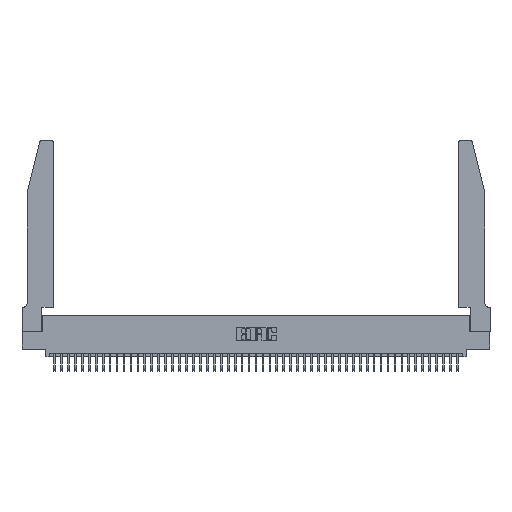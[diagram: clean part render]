
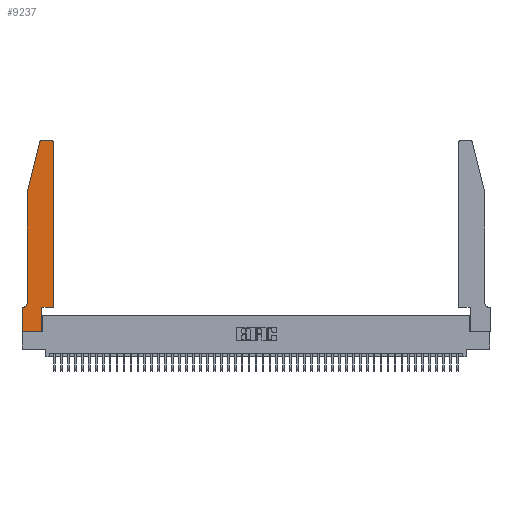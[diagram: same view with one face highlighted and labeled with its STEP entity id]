
A CAD part, top view. The second image highlights one B-rep face of the part: STEP entity #9237.
In plain terms, the highlighted planar face has unit normal (0, 0, 1).
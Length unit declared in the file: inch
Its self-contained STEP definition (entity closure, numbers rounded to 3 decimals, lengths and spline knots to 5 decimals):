
#523 = CARTESIAN_POINT ( 'NONE',  ( 0.25487, 2.72718, 0.37 ) ) ;
#570 = VECTOR ( 'NONE', #8482, 39.37008 ) ;
#900 = AXIS2_PLACEMENT_3D ( 'NONE', #37943, #14692, #41812 ) ;
#2733 = CARTESIAN_POINT ( 'NONE',  ( 0.2865, 0.35, 0.37 ) ) ;
#3807 = VERTEX_POINT ( 'NONE', #523 ) ;
#3835 = DIRECTION ( 'NONE',  ( -1., 0., 0. ) ) ;
#4139 = CARTESIAN_POINT ( 'NONE',  ( 0.4505, 0.35, 0.37 ) ) ;
#4190 = LINE ( 'NONE', #13538, #13559 ) ;
#4255 = VECTOR ( 'NONE', #35476, 39.37008 ) ;
#4504 = CARTESIAN_POINT ( 'NONE',  ( 0.4505, 0.35, 0.37 ) ) ;
#4843 = VERTEX_POINT ( 'NONE', #14845 ) ;
#5137 = VECTOR ( 'NONE', #28083, 39.37008 ) ;
#5609 = CARTESIAN_POINT ( 'NONE',  ( 0.4505, 0.35, 0.37 ) ) ;
#5718 = ORIENTED_EDGE ( 'NONE', *, *, #21342, .T. ) ;
#6091 = ORIENTED_EDGE ( 'NONE', *, *, #48705, .T. ) ;
#7346 = ORIENTED_EDGE ( 'NONE', *, *, #49079, .T. ) ;
#7571 = VERTEX_POINT ( 'NONE', #31948 ) ;
#7630 = LINE ( 'NONE', #24182, #5137 ) ;
#8482 = DIRECTION ( 'NONE',  ( 1., 0., 0. ) ) ;
#8710 = VERTEX_POINT ( 'NONE', #35243 ) ;
#9077 = AXIS2_PLACEMENT_3D ( 'NONE', #9098, #36387, #13149 ) ;
#9098 = CARTESIAN_POINT ( 'NONE',  ( 0.284, 2.72, 0.37 ) ) ;
#9120 = CARTESIAN_POINT ( 'NONE',  ( 0.0755, 0.42, 0.37 ) ) ;
#9237 = ADVANCED_FACE ( 'NONE', ( #25366 ), #18912, .T. ) ;
#9412 = CARTESIAN_POINT ( 'NONE',  ( 0.4205, 2.75, 0.37 ) ) ;
#9503 = DIRECTION ( 'NONE',  ( 0., -1., 0. ) ) ;
#10931 = DIRECTION ( 'NONE',  ( 0., -1., 0. ) ) ;
#11436 = LINE ( 'NONE', #42017, #29706 ) ;
#11728 = VERTEX_POINT ( 'NONE', #36708 ) ;
#12192 = CARTESIAN_POINT ( 'NONE',  ( 0.0755, 2., 0.37 ) ) ;
#13038 = ORIENTED_EDGE ( 'NONE', *, *, #16557, .T. ) ;
#13149 = DIRECTION ( 'NONE',  ( 1., 0., 0. ) ) ;
#13199 = ORIENTED_EDGE ( 'NONE', *, *, #35500, .T. ) ;
#13538 = CARTESIAN_POINT ( 'NONE',  ( 0.0755, 2., 0.37 ) ) ;
#13559 = VECTOR ( 'NONE', #9503, 39.37008 ) ;
#13911 = VERTEX_POINT ( 'NONE', #4139 ) ;
#14692 = DIRECTION ( 'NONE',  ( 0., 0., 1. ) ) ;
#14845 = CARTESIAN_POINT ( 'NONE',  ( 0.0055, 0.35, 0.37 ) ) ;
#15252 = CARTESIAN_POINT ( 'NONE',  ( 0.2605, 2.75, 0.37 ) ) ;
#15541 = ORIENTED_EDGE ( 'NONE', *, *, #18041, .T. ) ;
#15778 = LINE ( 'NONE', #5609, #24874 ) ;
#16062 = AXIS2_PLACEMENT_3D ( 'NONE', #50529, #27333, #3835 ) ;
#16424 = CARTESIAN_POINT ( 'NONE',  ( 0.2865, 0.35, 0.37 ) ) ;
#16557 = EDGE_CURVE ( 'NONE', #35021, #7571, #48352, .T. ) ;
#18041 = EDGE_CURVE ( 'NONE', #3807, #48240, #35471, .T. ) ;
#18402 = ORIENTED_EDGE ( 'NONE', *, *, #43440, .T. ) ;
#18912 = PLANE ( 'NONE',  #34100 ) ;
#19835 = CARTESIAN_POINT ( 'NONE',  ( 0.0755, 0.35, 0.37 ) ) ;
#20104 = ORIENTED_EDGE ( 'NONE', *, *, #31618, .T. ) ;
#20647 = LINE ( 'NONE', #19835, #32198 ) ;
#20684 = ORIENTED_EDGE ( 'NONE', *, *, #29722, .T. ) ;
#21342 = EDGE_CURVE ( 'NONE', #4843, #48756, #20647, .T. ) ;
#21578 = LINE ( 'NONE', #4504, #570 ) ;
#22808 = CIRCLE ( 'NONE', #9077, 0.03 ) ;
#22816 = DIRECTION ( 'NONE',  ( 0., 0., 1. ) ) ;
#24182 = CARTESIAN_POINT ( 'NONE',  ( 0., 0., 0.37 ) ) ;
#24226 = EDGE_CURVE ( 'NONE', #13911, #11728, #15778, .T. ) ;
#24404 = DIRECTION ( 'NONE',  ( 0., 1., 0. ) ) ;
#24874 = VECTOR ( 'NONE', #44471, 39.37008 ) ;
#25093 = EDGE_CURVE ( 'NONE', #44984, #8710, #7630, .T. ) ;
#25366 = FACE_OUTER_BOUND ( 'NONE', #36503, .T. ) ;
#27333 = DIRECTION ( 'NONE',  ( 0., 0., -1. ) ) ;
#28013 = ORIENTED_EDGE ( 'NONE', *, *, #32917, .T. ) ;
#28083 = DIRECTION ( 'NONE',  ( 1., 0., 0. ) ) ;
#29706 = VECTOR ( 'NONE', #10931, 39.37008 ) ;
#29722 = EDGE_CURVE ( 'NONE', #48756, #44984, #11436, .T. ) ;
#30852 = ORIENTED_EDGE ( 'NONE', *, *, #24226, .T. ) ;
#31618 = EDGE_CURVE ( 'NONE', #7571, #3807, #22808, .T. ) ;
#31948 = CARTESIAN_POINT ( 'NONE',  ( 0.284, 2.75, 0.37 ) ) ;
#32138 = ORIENTED_EDGE ( 'NONE', *, *, #25093, .T. ) ;
#32198 = VECTOR ( 'NONE', #46953, 39.37008 ) ;
#32917 = EDGE_CURVE ( 'NONE', #48240, #44332, #4190, .T. ) ;
#33121 = CARTESIAN_POINT ( 'NONE',  ( 0.0755, 2., 0.37 ) ) ;
#34032 = VERTEX_POINT ( 'NONE', #2733 ) ;
#34100 = AXIS2_PLACEMENT_3D ( 'NONE', #46015, #22816, #49908 ) ;
#34793 = VECTOR ( 'NONE', #24404, 39.37008 ) ;
#35021 = VERTEX_POINT ( 'NONE', #9412 ) ;
#35243 = CARTESIAN_POINT ( 'NONE',  ( 0.2865, 0., 0.37 ) ) ;
#35471 = LINE ( 'NONE', #12192, #4255 ) ;
#35476 = DIRECTION ( 'NONE',  ( -0.239, -0.971, 0. ) ) ;
#35500 = EDGE_CURVE ( 'NONE', #34032, #13911, #21578, .T. ) ;
#36064 = CARTESIAN_POINT ( 'NONE',  ( 0., 0., 0.37 ) ) ;
#36387 = DIRECTION ( 'NONE',  ( 0., 0., 1. ) ) ;
#36503 = EDGE_LOOP ( 'NONE', ( #13038, #20104, #15541, #28013, #18402, #5718, #20684, #32138, #6091, #13199, #30852, #7346 ) ) ;
#36708 = CARTESIAN_POINT ( 'NONE',  ( 0.4505, 2.72, 0.37 ) ) ;
#37943 = CARTESIAN_POINT ( 'NONE',  ( 0.4205, 2.72, 0.37 ) ) ;
#38622 = CIRCLE ( 'NONE', #16062, 0.07 ) ;
#40798 = CIRCLE ( 'NONE', #900, 0.03 ) ;
#41812 = DIRECTION ( 'NONE',  ( 1., 0., 0. ) ) ;
#42017 = CARTESIAN_POINT ( 'NONE',  ( 0., 0., 0.37 ) ) ;
#42197 = DIRECTION ( 'NONE',  ( -1., 0., 0. ) ) ;
#43440 = EDGE_CURVE ( 'NONE', #44332, #4843, #38622, .T. ) ;
#43872 = CARTESIAN_POINT ( 'NONE',  ( 0., 0.35, 0.37 ) ) ;
#44332 = VERTEX_POINT ( 'NONE', #9120 ) ;
#44471 = DIRECTION ( 'NONE',  ( 0., 1., 0. ) ) ;
#44984 = VERTEX_POINT ( 'NONE', #36064 ) ;
#46015 = CARTESIAN_POINT ( 'NONE',  ( 0., 0.35, 0.37 ) ) ;
#46290 = LINE ( 'NONE', #16424, #34793 ) ;
#46953 = DIRECTION ( 'NONE',  ( -1., 0., 0. ) ) ;
#47129 = VECTOR ( 'NONE', #42197, 39.37008 ) ;
#48240 = VERTEX_POINT ( 'NONE', #33121 ) ;
#48352 = LINE ( 'NONE', #15252, #47129 ) ;
#48705 = EDGE_CURVE ( 'NONE', #8710, #34032, #46290, .T. ) ;
#48756 = VERTEX_POINT ( 'NONE', #43872 ) ;
#49079 = EDGE_CURVE ( 'NONE', #11728, #35021, #40798, .T. ) ;
#49908 = DIRECTION ( 'NONE',  ( 1., 0., 0. ) ) ;
#50529 = CARTESIAN_POINT ( 'NONE',  ( 0.0055, 0.42, 0.37 ) ) ;
